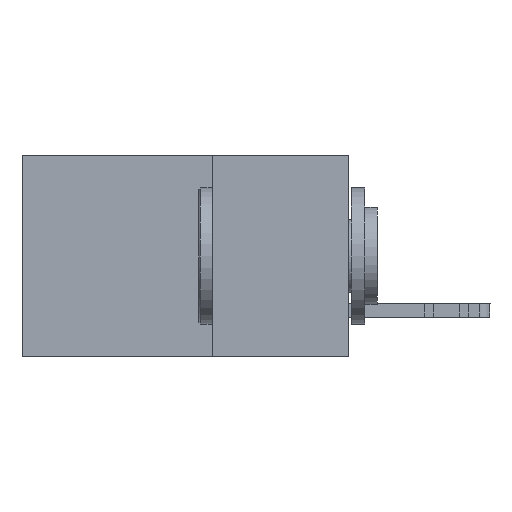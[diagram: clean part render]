
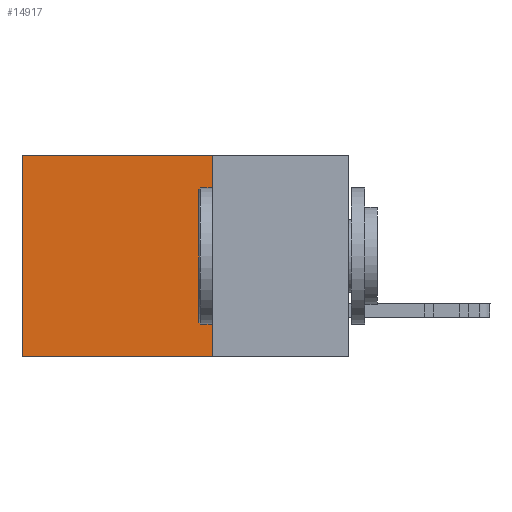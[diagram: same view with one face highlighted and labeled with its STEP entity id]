
A CAD part, left-side view. The second image highlights one B-rep face of the part: STEP entity #14917.
In plain terms, the highlighted planar face has unit normal (-1, 0, 0).
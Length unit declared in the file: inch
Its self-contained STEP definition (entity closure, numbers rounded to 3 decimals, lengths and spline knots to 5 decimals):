
#205 = VECTOR ( 'NONE', #2695, 39.37008 ) ;
#266 = LINE ( 'NONE', #3519, #13403 ) ;
#1149 = PLANE ( 'NONE',  #4138 ) ;
#1714 = ORIENTED_EDGE ( 'NONE', *, *, #3921, .F. ) ;
#1887 = DIRECTION ( 'NONE',  ( 0., 0., -1. ) ) ;
#1909 = DIRECTION ( 'NONE',  ( 0., 0., -1. ) ) ;
#2695 = DIRECTION ( 'NONE',  ( 0., 1., 0. ) ) ;
#2896 = FACE_OUTER_BOUND ( 'NONE', #20756, .T. ) ;
#3519 = CARTESIAN_POINT ( 'NONE',  ( 0.2615, 0.6, -0.37 ) ) ;
#3921 = EDGE_CURVE ( 'NONE', #14437, #9056, #14436, .T. ) ;
#4138 = AXIS2_PLACEMENT_3D ( 'NONE', #15316, #4744, #22381 ) ;
#4744 = DIRECTION ( 'NONE',  ( 1., 0., 0. ) ) ;
#5020 = EDGE_CURVE ( 'NONE', #9056, #9435, #20555, .T. ) ;
#6732 = ORIENTED_EDGE ( 'NONE', *, *, #14055, .T. ) ;
#7114 = CARTESIAN_POINT ( 'NONE',  ( 0.2615, 0.25, 0. ) ) ;
#8675 = CARTESIAN_POINT ( 'NONE',  ( 0.2615, 0.25, -0.37 ) ) ;
#9056 = VERTEX_POINT ( 'NONE', #8675 ) ;
#9435 = VERTEX_POINT ( 'NONE', #20933 ) ;
#11862 = CARTESIAN_POINT ( 'NONE',  ( 0.2615, 0.25, -0.37 ) ) ;
#12648 = VERTEX_POINT ( 'NONE', #17896 ) ;
#13403 = VECTOR ( 'NONE', #1887, 39.37008 ) ;
#14055 = EDGE_CURVE ( 'NONE', #12648, #9435, #266, .T. ) ;
#14436 = LINE ( 'NONE', #21510, #17750 ) ;
#14437 = VERTEX_POINT ( 'NONE', #20668 ) ;
#14917 = ADVANCED_FACE ( 'NONE', ( #2896 ), #1149, .F. ) ;
#15316 = CARTESIAN_POINT ( 'NONE',  ( 0.2615, 0.25, -0.37 ) ) ;
#16221 = ORIENTED_EDGE ( 'NONE', *, *, #21672, .T. ) ;
#17672 = LINE ( 'NONE', #7114, #19583 ) ;
#17750 = VECTOR ( 'NONE', #1909, 39.37008 ) ;
#17896 = CARTESIAN_POINT ( 'NONE',  ( 0.2615, 0.6, 0. ) ) ;
#19583 = VECTOR ( 'NONE', #21255, 39.37008 ) ;
#20145 = ORIENTED_EDGE ( 'NONE', *, *, #5020, .F. ) ;
#20555 = LINE ( 'NONE', #11862, #205 ) ;
#20668 = CARTESIAN_POINT ( 'NONE',  ( 0.2615, 0.25, 0. ) ) ;
#20756 = EDGE_LOOP ( 'NONE', ( #6732, #20145, #1714, #16221 ) ) ;
#20933 = CARTESIAN_POINT ( 'NONE',  ( 0.2615, 0.6, -0.37 ) ) ;
#21255 = DIRECTION ( 'NONE',  ( 0., 1., 0. ) ) ;
#21510 = CARTESIAN_POINT ( 'NONE',  ( 0.2615, 0.25, -0.37 ) ) ;
#21672 = EDGE_CURVE ( 'NONE', #14437, #12648, #17672, .T. ) ;
#22381 = DIRECTION ( 'NONE',  ( 0., 0., -1. ) ) ;
